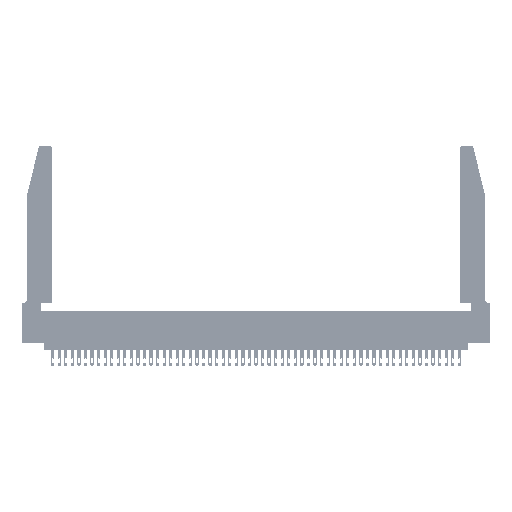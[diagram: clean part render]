
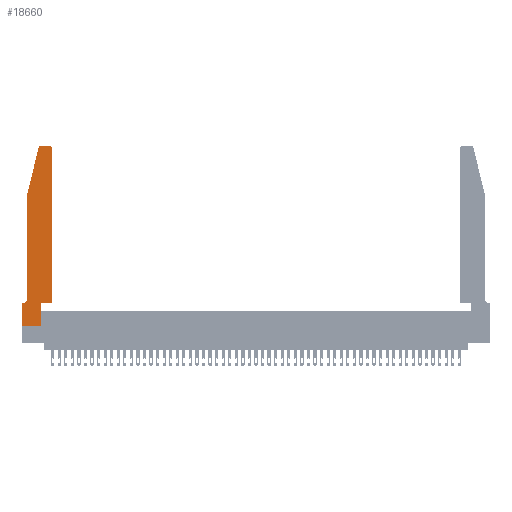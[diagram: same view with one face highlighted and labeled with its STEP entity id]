
A CAD part, top view. The second image highlights one B-rep face of the part: STEP entity #18660.
In plain terms, the highlighted planar face has unit normal (0, 0, 1).
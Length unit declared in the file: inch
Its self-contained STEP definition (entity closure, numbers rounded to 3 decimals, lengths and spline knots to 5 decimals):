
#352 = CARTESIAN_POINT ( 'NONE',  ( 0.0055, 0.42, 0.37 ) ) ;
#359 = CARTESIAN_POINT ( 'NONE',  ( 0., 0., 0.37 ) ) ;
#752 = VERTEX_POINT ( 'NONE', #45100 ) ;
#961 = ORIENTED_EDGE ( 'NONE', *, *, #4242, .T. ) ;
#1312 = VECTOR ( 'NONE', #30539, 39.37008 ) ;
#1385 = ORIENTED_EDGE ( 'NONE', *, *, #37368, .T. ) ;
#2606 = CARTESIAN_POINT ( 'NONE',  ( 0.0755, 0.42, 0.37 ) ) ;
#2756 = CARTESIAN_POINT ( 'NONE',  ( 0.4205, 2.72, 0.37 ) ) ;
#2980 = CARTESIAN_POINT ( 'NONE',  ( 0.0755, 2., 0.37 ) ) ;
#3381 = CARTESIAN_POINT ( 'NONE',  ( 0.25487, 2.72718, 0.37 ) ) ;
#4102 = VERTEX_POINT ( 'NONE', #18916 ) ;
#4242 = EDGE_CURVE ( 'NONE', #33797, #7903, #18853, .T. ) ;
#4301 = ORIENTED_EDGE ( 'NONE', *, *, #19539, .T. ) ;
#5333 = DIRECTION ( 'NONE',  ( 1., 0., 0. ) ) ;
#5400 = CARTESIAN_POINT ( 'NONE',  ( 0.2605, 2.75, 0.37 ) ) ;
#5470 = VECTOR ( 'NONE', #50578, 39.37008 ) ;
#5553 = CARTESIAN_POINT ( 'NONE',  ( 0.4505, 0.35, 0.37 ) ) ;
#5767 = CARTESIAN_POINT ( 'NONE',  ( 0.4205, 2.75, 0.37 ) ) ;
#5888 = CARTESIAN_POINT ( 'NONE',  ( 0.0755, 0.35, 0.37 ) ) ;
#6343 = AXIS2_PLACEMENT_3D ( 'NONE', #352, #32673, #17194 ) ;
#6386 = VERTEX_POINT ( 'NONE', #6511 ) ;
#6511 = CARTESIAN_POINT ( 'NONE',  ( 0.0055, 0.35, 0.37 ) ) ;
#6723 = DIRECTION ( 'NONE',  ( 0., 0., 1. ) ) ;
#7790 = EDGE_CURVE ( 'NONE', #26188, #14622, #39237, .T. ) ;
#7833 = VERTEX_POINT ( 'NONE', #2606 ) ;
#7903 = VERTEX_POINT ( 'NONE', #10535 ) ;
#8229 = VECTOR ( 'NONE', #17555, 39.37008 ) ;
#8432 = CARTESIAN_POINT ( 'NONE',  ( 0., 0., 0.37 ) ) ;
#9719 = CIRCLE ( 'NONE', #15126, 0.03 ) ;
#10535 = CARTESIAN_POINT ( 'NONE',  ( 0.284, 2.75, 0.37 ) ) ;
#11033 = AXIS2_PLACEMENT_3D ( 'NONE', #2756, #6723, #22691 ) ;
#13944 = DIRECTION ( 'NONE',  ( 0., -1., 0. ) ) ;
#14019 = LINE ( 'NONE', #42684, #46949 ) ;
#14622 = VERTEX_POINT ( 'NONE', #47140 ) ;
#15093 = DIRECTION ( 'NONE',  ( -0.239, -0.971, 0. ) ) ;
#15126 = AXIS2_PLACEMENT_3D ( 'NONE', #31146, #19809, #19638 ) ;
#15367 = EDGE_CURVE ( 'NONE', #7833, #6386, #35738, .T. ) ;
#16154 = VERTEX_POINT ( 'NONE', #28436 ) ;
#16207 = FACE_OUTER_BOUND ( 'NONE', #22593, .T. ) ;
#16341 = ORIENTED_EDGE ( 'NONE', *, *, #15367, .T. ) ;
#16772 = CARTESIAN_POINT ( 'NONE',  ( 0., 0.35, 0.37 ) ) ;
#17032 = AXIS2_PLACEMENT_3D ( 'NONE', #16772, #48572, #5333 ) ;
#17194 = DIRECTION ( 'NONE',  ( -1., 0., 0. ) ) ;
#17253 = LINE ( 'NONE', #22422, #5470 ) ;
#17555 = DIRECTION ( 'NONE',  ( -1., 0., 0. ) ) ;
#17922 = EDGE_CURVE ( 'NONE', #14622, #33797, #49905, .T. ) ;
#18351 = ORIENTED_EDGE ( 'NONE', *, *, #7790, .T. ) ;
#18627 = ORIENTED_EDGE ( 'NONE', *, *, #17922, .T. ) ;
#18660 = ADVANCED_FACE ( 'NONE', ( #16207 ), #40564, .T. ) ;
#18853 = LINE ( 'NONE', #5400, #8229 ) ;
#18916 = CARTESIAN_POINT ( 'NONE',  ( 0.2865, 0., 0.37 ) ) ;
#19532 = VECTOR ( 'NONE', #13944, 39.37008 ) ;
#19539 = EDGE_CURVE ( 'NONE', #4102, #36439, #26039, .T. ) ;
#19638 = DIRECTION ( 'NONE',  ( 1., 0., 0. ) ) ;
#19809 = DIRECTION ( 'NONE',  ( 0., 0., 1. ) ) ;
#22422 = CARTESIAN_POINT ( 'NONE',  ( 0.4505, 0.35, 0.37 ) ) ;
#22581 = EDGE_CURVE ( 'NONE', #16154, #49335, #14019, .T. ) ;
#22593 = EDGE_LOOP ( 'NONE', ( #961, #46583, #42911, #25161, #16341, #1385, #34417, #39251, #4301, #25379, #18351, #18627 ) ) ;
#22691 = DIRECTION ( 'NONE',  ( 1., 0., 0. ) ) ;
#24212 = CARTESIAN_POINT ( 'NONE',  ( 0.2865, 0.35, 0.37 ) ) ;
#24297 = CARTESIAN_POINT ( 'NONE',  ( 0.2865, 0.35, 0.37 ) ) ;
#25161 = ORIENTED_EDGE ( 'NONE', *, *, #51425, .T. ) ;
#25379 = ORIENTED_EDGE ( 'NONE', *, *, #34008, .T. ) ;
#26039 = LINE ( 'NONE', #24212, #42875 ) ;
#26188 = VERTEX_POINT ( 'NONE', #5553 ) ;
#26850 = CARTESIAN_POINT ( 'NONE',  ( 0.4505, 0.35, 0.37 ) ) ;
#27486 = EDGE_CURVE ( 'NONE', #49335, #4102, #29948, .T. ) ;
#27490 = VECTOR ( 'NONE', #49314, 39.37008 ) ;
#27716 = DIRECTION ( 'NONE',  ( 0., 1., 0. ) ) ;
#28128 = DIRECTION ( 'NONE',  ( 1., 0., 0. ) ) ;
#28436 = CARTESIAN_POINT ( 'NONE',  ( 0., 0.35, 0.37 ) ) ;
#29335 = VECTOR ( 'NONE', #28128, 39.37008 ) ;
#29948 = LINE ( 'NONE', #359, #29335 ) ;
#30539 = DIRECTION ( 'NONE',  ( 0., 1., 0. ) ) ;
#31146 = CARTESIAN_POINT ( 'NONE',  ( 0.284, 2.72, 0.37 ) ) ;
#32673 = DIRECTION ( 'NONE',  ( 0., 0., -1. ) ) ;
#33797 = VERTEX_POINT ( 'NONE', #5767 ) ;
#34008 = EDGE_CURVE ( 'NONE', #36439, #26188, #17253, .T. ) ;
#34417 = ORIENTED_EDGE ( 'NONE', *, *, #22581, .T. ) ;
#35738 = CIRCLE ( 'NONE', #6343, 0.07 ) ;
#36439 = VERTEX_POINT ( 'NONE', #24297 ) ;
#37368 = EDGE_CURVE ( 'NONE', #6386, #16154, #38132, .T. ) ;
#37428 = LINE ( 'NONE', #2980, #50509 ) ;
#37762 = CARTESIAN_POINT ( 'NONE',  ( 0.0755, 2., 0.37 ) ) ;
#38132 = LINE ( 'NONE', #5888, #27490 ) ;
#39237 = LINE ( 'NONE', #26850, #1312 ) ;
#39251 = ORIENTED_EDGE ( 'NONE', *, *, #27486, .T. ) ;
#39845 = DIRECTION ( 'NONE',  ( 0., -1., 0. ) ) ;
#39882 = VERTEX_POINT ( 'NONE', #3381 ) ;
#40019 = EDGE_CURVE ( 'NONE', #7903, #39882, #9719, .T. ) ;
#40564 = PLANE ( 'NONE',  #17032 ) ;
#42684 = CARTESIAN_POINT ( 'NONE',  ( 0., 0., 0.37 ) ) ;
#42875 = VECTOR ( 'NONE', #27716, 39.37008 ) ;
#42911 = ORIENTED_EDGE ( 'NONE', *, *, #43435, .T. ) ;
#43181 = LINE ( 'NONE', #37762, #19532 ) ;
#43435 = EDGE_CURVE ( 'NONE', #39882, #752, #37428, .T. ) ;
#45100 = CARTESIAN_POINT ( 'NONE',  ( 0.0755, 2., 0.37 ) ) ;
#46583 = ORIENTED_EDGE ( 'NONE', *, *, #40019, .T. ) ;
#46949 = VECTOR ( 'NONE', #39845, 39.37008 ) ;
#47140 = CARTESIAN_POINT ( 'NONE',  ( 0.4505, 2.72, 0.37 ) ) ;
#48572 = DIRECTION ( 'NONE',  ( 0., 0., 1. ) ) ;
#49314 = DIRECTION ( 'NONE',  ( -1., 0., 0. ) ) ;
#49335 = VERTEX_POINT ( 'NONE', #8432 ) ;
#49905 = CIRCLE ( 'NONE', #11033, 0.03 ) ;
#50509 = VECTOR ( 'NONE', #15093, 39.37008 ) ;
#50578 = DIRECTION ( 'NONE',  ( 1., 0., 0. ) ) ;
#51425 = EDGE_CURVE ( 'NONE', #752, #7833, #43181, .T. ) ;
